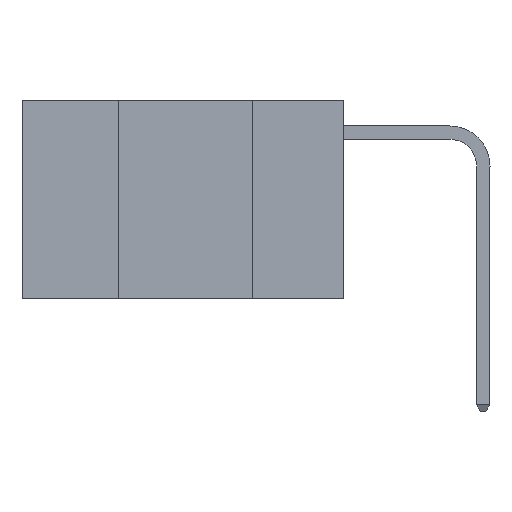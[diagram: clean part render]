
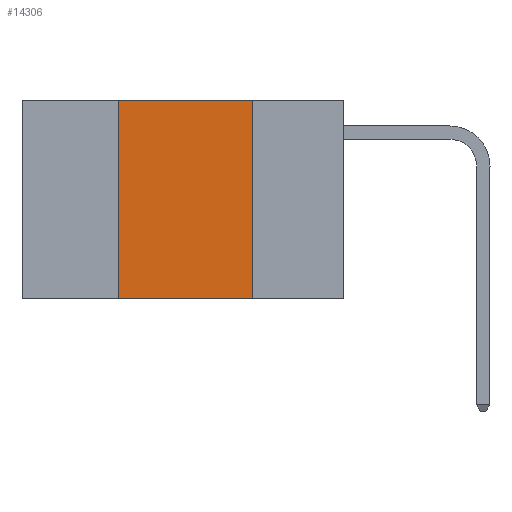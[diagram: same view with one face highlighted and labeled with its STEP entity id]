
A CAD part, left-side view. The second image highlights one B-rep face of the part: STEP entity #14306.
In plain terms, the highlighted planar face has unit normal (-1, 0, 0).
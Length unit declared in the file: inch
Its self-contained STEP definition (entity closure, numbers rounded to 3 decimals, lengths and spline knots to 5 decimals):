
#129 = VERTEX_POINT ( 'NONE', #14028 ) ;
#402 = FACE_OUTER_BOUND ( 'NONE', #7914, .T. ) ;
#634 = DIRECTION ( 'NONE',  ( 0., -1., 0. ) ) ;
#846 = VECTOR ( 'NONE', #15812, 39.37008 ) ;
#953 = CARTESIAN_POINT ( 'NONE',  ( 0., 0.42, 0. ) ) ;
#1497 = ORIENTED_EDGE ( 'NONE', *, *, #13286, .F. ) ;
#1990 = CARTESIAN_POINT ( 'NONE',  ( 0., 0.6, 0. ) ) ;
#2295 = DIRECTION ( 'NONE',  ( 0., -1., 0. ) ) ;
#3408 = VECTOR ( 'NONE', #634, 39.37008 ) ;
#4148 = EDGE_CURVE ( 'NONE', #7101, #13592, #14503, .T. ) ;
#4488 = DIRECTION ( 'NONE',  ( 0., 0., -1. ) ) ;
#4533 = LINE ( 'NONE', #7449, #10772 ) ;
#4823 = ORIENTED_EDGE ( 'NONE', *, *, #5013, .F. ) ;
#5013 = EDGE_CURVE ( 'NONE', #7101, #11814, #7469, .T. ) ;
#5828 = EDGE_CURVE ( 'NONE', #129, #13592, #4533, .T. ) ;
#7101 = VERTEX_POINT ( 'NONE', #9757 ) ;
#7320 = ORIENTED_EDGE ( 'NONE', *, *, #5828, .F. ) ;
#7449 = CARTESIAN_POINT ( 'NONE',  ( 0., 0.17, 0. ) ) ;
#7469 = LINE ( 'NONE', #953, #846 ) ;
#7809 = CARTESIAN_POINT ( 'NONE',  ( 0., 0.17, -0.37 ) ) ;
#7914 = EDGE_LOOP ( 'NONE', ( #7320, #1497, #4823, #8512 ) ) ;
#8486 = CARTESIAN_POINT ( 'NONE',  ( 0., 0.6, 0. ) ) ;
#8512 = ORIENTED_EDGE ( 'NONE', *, *, #4148, .T. ) ;
#8721 = DIRECTION ( 'NONE',  ( 0., 0., -1. ) ) ;
#9443 = PLANE ( 'NONE',  #11950 ) ;
#9757 = CARTESIAN_POINT ( 'NONE',  ( 0., 0.42, -0.37 ) ) ;
#10772 = VECTOR ( 'NONE', #8721, 39.37008 ) ;
#11814 = VERTEX_POINT ( 'NONE', #12787 ) ;
#11950 = AXIS2_PLACEMENT_3D ( 'NONE', #1990, #11981, #4488 ) ;
#11981 = DIRECTION ( 'NONE',  ( 1., 0., 0. ) ) ;
#12396 = VECTOR ( 'NONE', #2295, 39.37008 ) ;
#12787 = CARTESIAN_POINT ( 'NONE',  ( 0., 0.42, 0. ) ) ;
#13286 = EDGE_CURVE ( 'NONE', #11814, #129, #15989, .T. ) ;
#13592 = VERTEX_POINT ( 'NONE', #7809 ) ;
#14028 = CARTESIAN_POINT ( 'NONE',  ( 0., 0.17, 0. ) ) ;
#14306 = ADVANCED_FACE ( 'NONE', ( #402 ), #9443, .F. ) ;
#14503 = LINE ( 'NONE', #15508, #3408 ) ;
#15508 = CARTESIAN_POINT ( 'NONE',  ( 0., 0.6, -0.37 ) ) ;
#15812 = DIRECTION ( 'NONE',  ( 0., 0., 1. ) ) ;
#15989 = LINE ( 'NONE', #8486, #12396 ) ;
